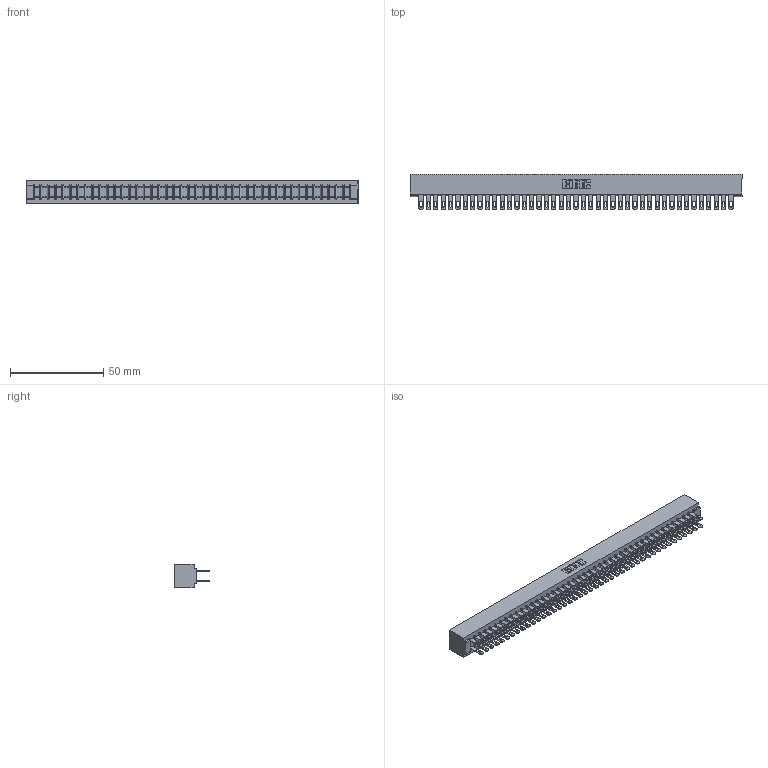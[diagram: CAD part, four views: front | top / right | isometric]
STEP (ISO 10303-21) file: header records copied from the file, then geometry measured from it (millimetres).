
FILE_DESCRIPTION (( 'STEP AP203' ), '1' );
FILE_NAME ('357-086-400-201.STEP', '2020-10-04T07:07:59', ( '' ), ( '' ), 'SwSTEP 2.0', 'SolidWorks 2020', '' );
FILE_SCHEMA (( 'CONFIG_CONTROL_DESIGN' ));
Length unit declared in the file: inch
Products named in the file (3): 307 Part_No Mounting Lugs; 307-290-001_500; 357-086-400-201
Assembly tree (87 placements, depth 2):
  357-086-400-201
    307 Part_No Mounting Lugs
    307-290-001_500  x86
Bounding box: 178.26 x 19.18 x 12.7 mm (x, y, z)
Volume: 19756.6 mm3; surface area: 25877.1 mm2
Topology: 87 solids, 87 shells, 4110 faces, 11479 edges, 7418 vertices
Faces by surface type: plane 2646, cylinder 1376, sphere 88
Entity records: 37812 total; most frequent: CARTESIAN_POINT 6179, ORIENTED_EDGE 6122, DIRECTION 6053, EDGE_CURVE 3061, LINE 2349, VECTOR 2349, VERTEX_POINT 1978, AXIS2_PLACEMENT_3D 1852
